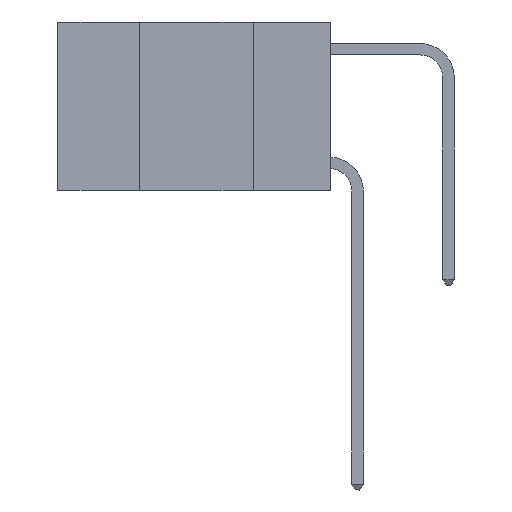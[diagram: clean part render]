
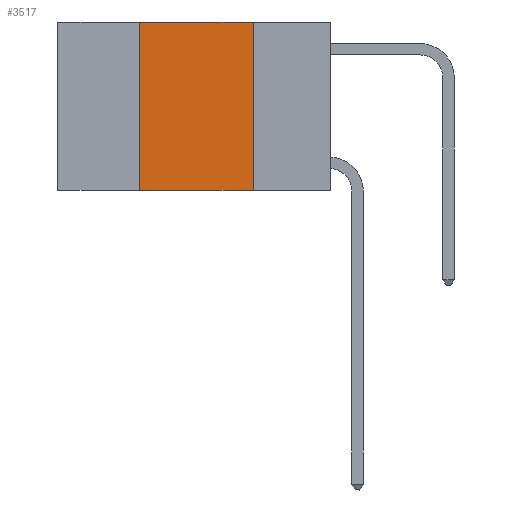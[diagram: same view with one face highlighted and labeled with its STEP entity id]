
A CAD part, left-side view. The second image highlights one B-rep face of the part: STEP entity #3517.
In plain terms, the highlighted planar face has unit normal (-1, 0, 0).
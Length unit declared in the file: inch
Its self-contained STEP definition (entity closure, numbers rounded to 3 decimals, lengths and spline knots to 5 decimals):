
#364 = ORIENTED_EDGE ( 'NONE', *, *, #4310, .F. ) ;
#977 = CARTESIAN_POINT ( 'NONE',  ( 0., 0.6, -0.37 ) ) ;
#1176 = VERTEX_POINT ( 'NONE', #3642 ) ;
#1260 = CARTESIAN_POINT ( 'NONE',  ( 0., 0.42, 0. ) ) ;
#1394 = VECTOR ( 'NONE', #3726, 39.37008 ) ;
#1712 = CARTESIAN_POINT ( 'NONE',  ( 0., 0.42, -0.37 ) ) ;
#1786 = VERTEX_POINT ( 'NONE', #8508 ) ;
#2006 = LINE ( 'NONE', #11289, #10960 ) ;
#2015 = VERTEX_POINT ( 'NONE', #1712 ) ;
#2701 = LINE ( 'NONE', #5490, #1394 ) ;
#2791 = EDGE_CURVE ( 'NONE', #2015, #1176, #6496, .T. ) ;
#3295 = VERTEX_POINT ( 'NONE', #1260 ) ;
#3517 = ADVANCED_FACE ( 'NONE', ( #4660 ), #11130, .F. ) ;
#3642 = CARTESIAN_POINT ( 'NONE',  ( 0., 0.17, -0.37 ) ) ;
#3726 = DIRECTION ( 'NONE',  ( 0., 0., 1. ) ) ;
#4243 = EDGE_LOOP ( 'NONE', ( #5249, #8844, #364, #5016 ) ) ;
#4310 = EDGE_CURVE ( 'NONE', #2015, #3295, #2701, .T. ) ;
#4660 = FACE_OUTER_BOUND ( 'NONE', #4243, .T. ) ;
#4707 = AXIS2_PLACEMENT_3D ( 'NONE', #6184, #11273, #8141 ) ;
#5016 = ORIENTED_EDGE ( 'NONE', *, *, #2791, .T. ) ;
#5249 = ORIENTED_EDGE ( 'NONE', *, *, #7987, .F. ) ;
#5266 = EDGE_CURVE ( 'NONE', #3295, #1786, #6727, .T. ) ;
#5490 = CARTESIAN_POINT ( 'NONE',  ( 0., 0.42, 0. ) ) ;
#5962 = DIRECTION ( 'NONE',  ( 0., 0., -1. ) ) ;
#6184 = CARTESIAN_POINT ( 'NONE',  ( 0., 0.6, 0. ) ) ;
#6496 = LINE ( 'NONE', #977, #7777 ) ;
#6727 = LINE ( 'NONE', #9673, #11030 ) ;
#7777 = VECTOR ( 'NONE', #11293, 39.37008 ) ;
#7987 = EDGE_CURVE ( 'NONE', #1786, #1176, #2006, .T. ) ;
#8141 = DIRECTION ( 'NONE',  ( 0., 0., -1. ) ) ;
#8508 = CARTESIAN_POINT ( 'NONE',  ( 0., 0.17, 0. ) ) ;
#8844 = ORIENTED_EDGE ( 'NONE', *, *, #5266, .F. ) ;
#9673 = CARTESIAN_POINT ( 'NONE',  ( 0., 0.6, 0. ) ) ;
#10960 = VECTOR ( 'NONE', #5962, 39.37008 ) ;
#11030 = VECTOR ( 'NONE', #11590, 39.37008 ) ;
#11130 = PLANE ( 'NONE',  #4707 ) ;
#11273 = DIRECTION ( 'NONE',  ( 1., 0., 0. ) ) ;
#11289 = CARTESIAN_POINT ( 'NONE',  ( 0., 0.17, 0. ) ) ;
#11293 = DIRECTION ( 'NONE',  ( 0., -1., 0. ) ) ;
#11590 = DIRECTION ( 'NONE',  ( 0., -1., 0. ) ) ;
